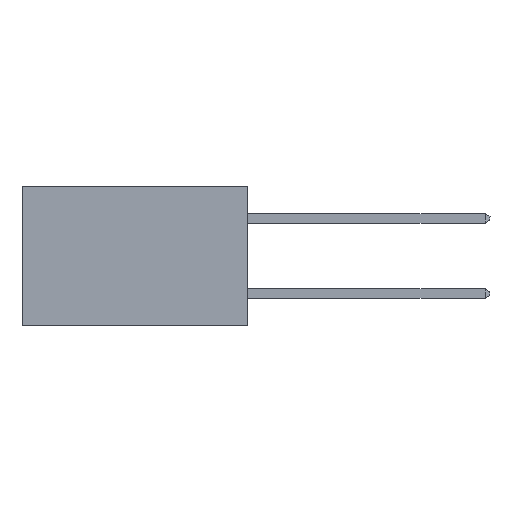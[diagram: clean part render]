
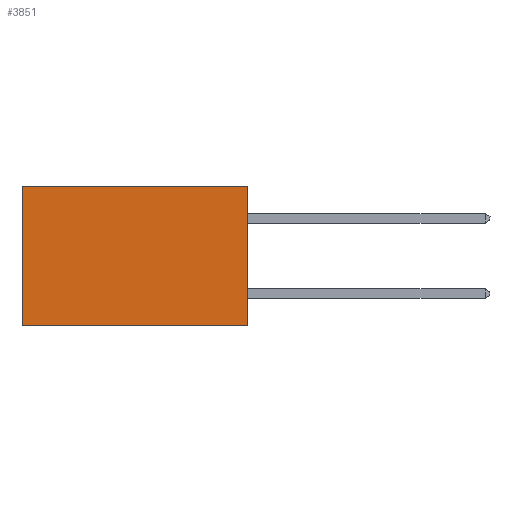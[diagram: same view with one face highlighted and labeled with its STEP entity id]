
A CAD part, left-side view. The second image highlights one B-rep face of the part: STEP entity #3851.
In plain terms, the highlighted planar face has unit normal (-1, 0, 0).
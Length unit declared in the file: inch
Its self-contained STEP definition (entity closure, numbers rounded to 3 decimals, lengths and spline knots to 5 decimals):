
#209 = CARTESIAN_POINT ( 'NONE',  ( 0.298, 0., -0.37 ) ) ;
#441 = FACE_OUTER_BOUND ( 'NONE', #8498, .T. ) ;
#768 = VECTOR ( 'NONE', #1973, 39.37008 ) ;
#1067 = VECTOR ( 'NONE', #3737, 39.37008 ) ;
#1383 = VERTEX_POINT ( 'NONE', #12771 ) ;
#1973 = DIRECTION ( 'NONE',  ( 0., 1., 0. ) ) ;
#2033 = AXIS2_PLACEMENT_3D ( 'NONE', #4534, #11462, #5511 ) ;
#2657 = CARTESIAN_POINT ( 'NONE',  ( 0.298, 0., -0.37 ) ) ;
#2976 = ORIENTED_EDGE ( 'NONE', *, *, #4133, .F. ) ;
#3710 = ORIENTED_EDGE ( 'NONE', *, *, #10359, .F. ) ;
#3737 = DIRECTION ( 'NONE',  ( 0., 0., -1. ) ) ;
#3851 = ADVANCED_FACE ( 'NONE', ( #441 ), #9465, .F. ) ;
#3878 = VECTOR ( 'NONE', #10824, 39.37008 ) ;
#4133 = EDGE_CURVE ( 'NONE', #1383, #6353, #11022, .T. ) ;
#4534 = CARTESIAN_POINT ( 'NONE',  ( 0.298, 0., 0. ) ) ;
#4710 = EDGE_CURVE ( 'NONE', #8983, #9047, #11843, .T. ) ;
#4724 = EDGE_CURVE ( 'NONE', #1383, #8983, #7751, .T. ) ;
#5511 = DIRECTION ( 'NONE',  ( 0., 0., -1. ) ) ;
#5856 = CARTESIAN_POINT ( 'NONE',  ( 0.298, 0.6, 0. ) ) ;
#6022 = CARTESIAN_POINT ( 'NONE',  ( 0.298, 0., 0. ) ) ;
#6353 = VERTEX_POINT ( 'NONE', #2657 ) ;
#7751 = LINE ( 'NONE', #6022, #768 ) ;
#7871 = LINE ( 'NONE', #209, #8501 ) ;
#8498 = EDGE_LOOP ( 'NONE', ( #11267, #3710, #2976, #11980 ) ) ;
#8501 = VECTOR ( 'NONE', #10197, 39.37008 ) ;
#8983 = VERTEX_POINT ( 'NONE', #10570 ) ;
#9047 = VERTEX_POINT ( 'NONE', #10687 ) ;
#9465 = PLANE ( 'NONE',  #2033 ) ;
#10197 = DIRECTION ( 'NONE',  ( 0., 1., 0. ) ) ;
#10359 = EDGE_CURVE ( 'NONE', #6353, #9047, #7871, .T. ) ;
#10570 = CARTESIAN_POINT ( 'NONE',  ( 0.298, 0.6, 0. ) ) ;
#10687 = CARTESIAN_POINT ( 'NONE',  ( 0.298, 0.6, -0.37 ) ) ;
#10824 = DIRECTION ( 'NONE',  ( 0., 0., -1. ) ) ;
#11022 = LINE ( 'NONE', #11742, #1067 ) ;
#11267 = ORIENTED_EDGE ( 'NONE', *, *, #4710, .T. ) ;
#11462 = DIRECTION ( 'NONE',  ( 1., 0., 0. ) ) ;
#11742 = CARTESIAN_POINT ( 'NONE',  ( 0.298, 0., 0. ) ) ;
#11843 = LINE ( 'NONE', #5856, #3878 ) ;
#11980 = ORIENTED_EDGE ( 'NONE', *, *, #4724, .T. ) ;
#12771 = CARTESIAN_POINT ( 'NONE',  ( 0.298, 0., 0. ) ) ;
